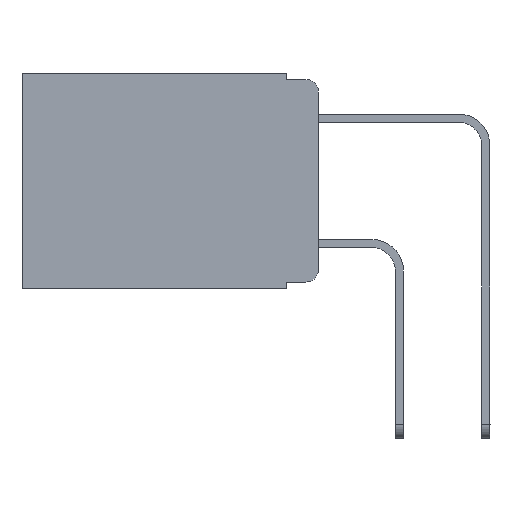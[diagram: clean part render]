
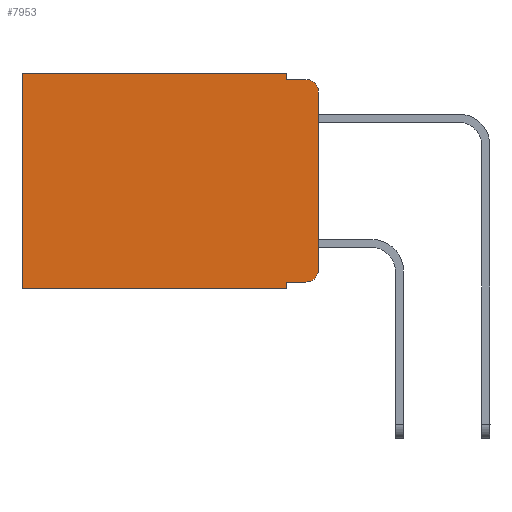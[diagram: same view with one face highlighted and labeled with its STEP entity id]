
A CAD part, left-side view. The second image highlights one B-rep face of the part: STEP entity #7953.
In plain terms, the highlighted planar face has unit normal (-1, 0, 0).
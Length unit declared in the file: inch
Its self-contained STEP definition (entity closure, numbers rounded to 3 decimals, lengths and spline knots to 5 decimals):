
#34 = FACE_OUTER_BOUND ( 'NONE', #785, .T. ) ;
#83 = VERTEX_POINT ( 'NONE', #5452 ) ;
#133 = LINE ( 'NONE', #4462, #8060 ) ;
#518 = CARTESIAN_POINT ( 'NONE',  ( 0.298, 0.051, 0. ) ) ;
#785 = EDGE_LOOP ( 'NONE', ( #13664, #3640, #12793, #1417, #4808, #10710, #6805, #13864, #6887, #10189 ) ) ;
#833 = EDGE_CURVE ( 'NONE', #6269, #3856, #10477, .T. ) ;
#882 = CARTESIAN_POINT ( 'NONE',  ( 0.298, 0.02, -0.333 ) ) ;
#963 = LINE ( 'NONE', #12735, #12052 ) ;
#1244 = DIRECTION ( 'NONE',  ( 0., 0., -1. ) ) ;
#1338 = CARTESIAN_POINT ( 'NONE',  ( 0.298, 0.02, -0.01 ) ) ;
#1417 = ORIENTED_EDGE ( 'NONE', *, *, #4710, .F. ) ;
#2121 = LINE ( 'NONE', #3048, #3369 ) ;
#2154 = EDGE_CURVE ( 'NONE', #7940, #3607, #963, .T. ) ;
#2165 = VECTOR ( 'NONE', #8936, 39.37008 ) ;
#2257 = CARTESIAN_POINT ( 'NONE',  ( 0.298, 0.051, -0.343 ) ) ;
#2457 = CARTESIAN_POINT ( 'NONE',  ( 0.298, 0., 0. ) ) ;
#2523 = DIRECTION ( 'NONE',  ( -1., 0., 0. ) ) ;
#2798 = CARTESIAN_POINT ( 'NONE',  ( 0.298, 0., -0.03 ) ) ;
#2879 = CARTESIAN_POINT ( 'NONE',  ( 0.298, 0., -0.313 ) ) ;
#3048 = CARTESIAN_POINT ( 'NONE',  ( 0.298, 0.051, 0. ) ) ;
#3138 = EDGE_CURVE ( 'NONE', #8036, #3186, #3561, .T. ) ;
#3186 = VERTEX_POINT ( 'NONE', #882 ) ;
#3215 = VECTOR ( 'NONE', #11846, 39.37008 ) ;
#3369 = VECTOR ( 'NONE', #10696, 39.37008 ) ;
#3561 = LINE ( 'NONE', #6602, #3215 ) ;
#3586 = EDGE_CURVE ( 'NONE', #9601, #3856, #4461, .T. ) ;
#3607 = VERTEX_POINT ( 'NONE', #1338 ) ;
#3640 = ORIENTED_EDGE ( 'NONE', *, *, #13713, .T. ) ;
#3856 = VERTEX_POINT ( 'NONE', #3893 ) ;
#3893 = CARTESIAN_POINT ( 'NONE',  ( 0.298, 0.473, -0.343 ) ) ;
#4461 = LINE ( 'NONE', #4535, #6512 ) ;
#4462 = CARTESIAN_POINT ( 'NONE',  ( 0.298, 0., 0. ) ) ;
#4535 = CARTESIAN_POINT ( 'NONE',  ( 0.298, 0.473, 0. ) ) ;
#4710 = EDGE_CURVE ( 'NONE', #83, #7940, #2121, .T. ) ;
#4808 = ORIENTED_EDGE ( 'NONE', *, *, #12370, .T. ) ;
#4832 = DIRECTION ( 'NONE',  ( 0., 0., -1. ) ) ;
#4907 = LINE ( 'NONE', #518, #5298 ) ;
#4944 = CARTESIAN_POINT ( 'NONE',  ( 0.298, 0., -0.343 ) ) ;
#5298 = VECTOR ( 'NONE', #4832, 39.37008 ) ;
#5452 = CARTESIAN_POINT ( 'NONE',  ( 0.298, 0.051, 0. ) ) ;
#5782 = AXIS2_PLACEMENT_3D ( 'NONE', #13540, #9220, #8960 ) ;
#5855 = CIRCLE ( 'NONE', #10845, 0.02 ) ;
#6269 = VERTEX_POINT ( 'NONE', #2257 ) ;
#6512 = VECTOR ( 'NONE', #10978, 39.37008 ) ;
#6602 = CARTESIAN_POINT ( 'NONE',  ( 0.298, 0.051, -0.333 ) ) ;
#6775 = CARTESIAN_POINT ( 'NONE',  ( 0.298, 0.051, -0.333 ) ) ;
#6805 = ORIENTED_EDGE ( 'NONE', *, *, #833, .F. ) ;
#6887 = ORIENTED_EDGE ( 'NONE', *, *, #3138, .T. ) ;
#6944 = EDGE_CURVE ( 'NONE', #3186, #8290, #5855, .T. ) ;
#7940 = VERTEX_POINT ( 'NONE', #8986 ) ;
#7953 = ADVANCED_FACE ( 'NONE', ( #34 ), #12163, .F. ) ;
#8036 = VERTEX_POINT ( 'NONE', #6775 ) ;
#8060 = VECTOR ( 'NONE', #9768, 39.37008 ) ;
#8287 = DIRECTION ( 'NONE',  ( 0., 1., 0. ) ) ;
#8290 = VERTEX_POINT ( 'NONE', #2879 ) ;
#8936 = DIRECTION ( 'NONE',  ( 0., 0., -1. ) ) ;
#8960 = DIRECTION ( 'NONE',  ( 0., 0., -1. ) ) ;
#8986 = CARTESIAN_POINT ( 'NONE',  ( 0.298, 0.051, -0.01 ) ) ;
#9220 = DIRECTION ( 'NONE',  ( -1., 0., 0. ) ) ;
#9601 = VERTEX_POINT ( 'NONE', #11938 ) ;
#9768 = DIRECTION ( 'NONE',  ( 0., 1., 0. ) ) ;
#9839 = CARTESIAN_POINT ( 'NONE',  ( 0.298, 0., 0. ) ) ;
#10189 = ORIENTED_EDGE ( 'NONE', *, *, #6944, .T. ) ;
#10352 = VECTOR ( 'NONE', #8287, 39.37008 ) ;
#10438 = EDGE_CURVE ( 'NONE', #8036, #6269, #4907, .T. ) ;
#10477 = LINE ( 'NONE', #4944, #10352 ) ;
#10696 = DIRECTION ( 'NONE',  ( 0., 0., -1. ) ) ;
#10710 = ORIENTED_EDGE ( 'NONE', *, *, #3586, .T. ) ;
#10817 = DIRECTION ( 'NONE',  ( 1., 0., 0. ) ) ;
#10845 = AXIS2_PLACEMENT_3D ( 'NONE', #11639, #2523, #11839 ) ;
#10865 = AXIS2_PLACEMENT_3D ( 'NONE', #2457, #10817, #1244 ) ;
#10978 = DIRECTION ( 'NONE',  ( 0., 0., -1. ) ) ;
#11611 = DIRECTION ( 'NONE',  ( 0., -1., 0. ) ) ;
#11639 = CARTESIAN_POINT ( 'NONE',  ( 0.298, 0.02, -0.313 ) ) ;
#11839 = DIRECTION ( 'NONE',  ( 0., 0., -1. ) ) ;
#11846 = DIRECTION ( 'NONE',  ( 0., -1., 0. ) ) ;
#11894 = CIRCLE ( 'NONE', #5782, 0.02 ) ;
#11938 = CARTESIAN_POINT ( 'NONE',  ( 0.298, 0.473, 0. ) ) ;
#12052 = VECTOR ( 'NONE', #11611, 39.37008 ) ;
#12163 = PLANE ( 'NONE',  #10865 ) ;
#12352 = EDGE_CURVE ( 'NONE', #13472, #8290, #13037, .T. ) ;
#12370 = EDGE_CURVE ( 'NONE', #83, #9601, #133, .T. ) ;
#12735 = CARTESIAN_POINT ( 'NONE',  ( 0.298, 0.051, -0.01 ) ) ;
#12793 = ORIENTED_EDGE ( 'NONE', *, *, #2154, .F. ) ;
#13037 = LINE ( 'NONE', #9839, #2165 ) ;
#13472 = VERTEX_POINT ( 'NONE', #2798 ) ;
#13540 = CARTESIAN_POINT ( 'NONE',  ( 0.298, 0.02, -0.03 ) ) ;
#13664 = ORIENTED_EDGE ( 'NONE', *, *, #12352, .F. ) ;
#13713 = EDGE_CURVE ( 'NONE', #13472, #3607, #11894, .T. ) ;
#13864 = ORIENTED_EDGE ( 'NONE', *, *, #10438, .F. ) ;
